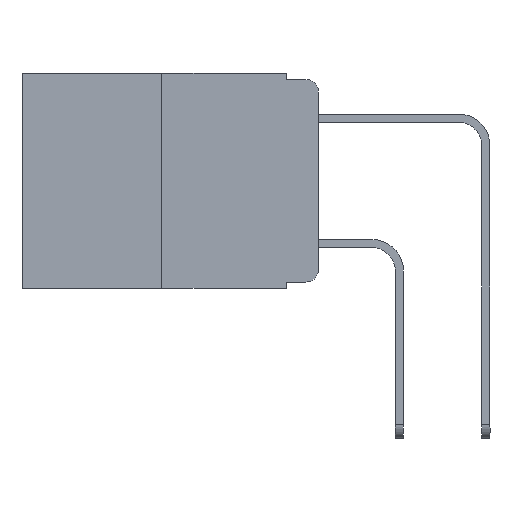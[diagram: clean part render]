
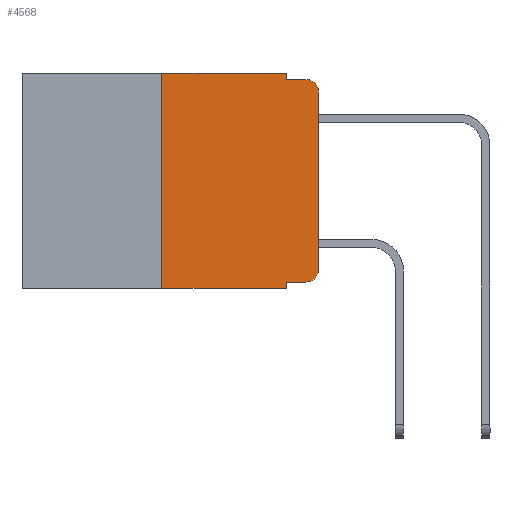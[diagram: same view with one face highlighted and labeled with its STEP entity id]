
A CAD part, left-side view. The second image highlights one B-rep face of the part: STEP entity #4568.
In plain terms, the highlighted planar face has unit normal (-1, 0, 0).
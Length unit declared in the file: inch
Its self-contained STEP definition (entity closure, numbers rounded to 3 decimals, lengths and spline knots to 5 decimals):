
#183 = ORIENTED_EDGE ( 'NONE', *, *, #6153, .F. ) ;
#1102 = CARTESIAN_POINT ( 'NONE',  ( 0., 0.051, -0.333 ) ) ;
#1154 = EDGE_CURVE ( 'NONE', #12393, #10170, #1194, .T. ) ;
#1194 = LINE ( 'NONE', #10466, #10949 ) ;
#1299 = DIRECTION ( 'NONE',  ( 0., 0., -1. ) ) ;
#1420 = ORIENTED_EDGE ( 'NONE', *, *, #4232, .T. ) ;
#1566 = FACE_OUTER_BOUND ( 'NONE', #10264, .T. ) ;
#1589 = AXIS2_PLACEMENT_3D ( 'NONE', #11448, #7667, #1299 ) ;
#1647 = CARTESIAN_POINT ( 'NONE',  ( 0., 0.02, -0.01 ) ) ;
#2068 = CARTESIAN_POINT ( 'NONE',  ( 0., 0.051, 0. ) ) ;
#2084 = EDGE_CURVE ( 'NONE', #12351, #12169, #6772, .T. ) ;
#2119 = VECTOR ( 'NONE', #5809, 39.37008 ) ;
#2302 = ORIENTED_EDGE ( 'NONE', *, *, #6197, .T. ) ;
#2323 = VECTOR ( 'NONE', #10333, 39.37008 ) ;
#2584 = ORIENTED_EDGE ( 'NONE', *, *, #8001, .T. ) ;
#2593 = DIRECTION ( 'NONE',  ( 0., 0., -1. ) ) ;
#2973 = ORIENTED_EDGE ( 'NONE', *, *, #6102, .T. ) ;
#3120 = CIRCLE ( 'NONE', #8015, 0.02 ) ;
#3357 = EDGE_CURVE ( 'NONE', #7927, #4158, #3972, .T. ) ;
#3972 = LINE ( 'NONE', #12029, #10428 ) ;
#4046 = VECTOR ( 'NONE', #10812, 39.37008 ) ;
#4158 = VERTEX_POINT ( 'NONE', #11807 ) ;
#4232 = EDGE_CURVE ( 'NONE', #13104, #12169, #13054, .T. ) ;
#4300 = DIRECTION ( 'NONE',  ( 0., 0., 1. ) ) ;
#4515 = CARTESIAN_POINT ( 'NONE',  ( 0., 0.051, -0.01 ) ) ;
#4538 = PLANE ( 'NONE',  #9386 ) ;
#4568 = ADVANCED_FACE ( 'NONE', ( #1566 ), #4538, .F. ) ;
#4780 = LINE ( 'NONE', #11014, #6780 ) ;
#5189 = DIRECTION ( 'NONE',  ( 0., -1., 0. ) ) ;
#5514 = CARTESIAN_POINT ( 'NONE',  ( 0., 0.02, -0.313 ) ) ;
#5528 = CARTESIAN_POINT ( 'NONE',  ( 0., 0.473, 0. ) ) ;
#5641 = ORIENTED_EDGE ( 'NONE', *, *, #3357, .F. ) ;
#5809 = DIRECTION ( 'NONE',  ( 0., -1., 0. ) ) ;
#5896 = CARTESIAN_POINT ( 'NONE',  ( 0., 0.051, -0.343 ) ) ;
#5912 = DIRECTION ( 'NONE',  ( 0., 0., 1. ) ) ;
#5971 = DIRECTION ( 'NONE',  ( 0., -1., 0. ) ) ;
#6089 = LINE ( 'NONE', #2068, #2323 ) ;
#6102 = EDGE_CURVE ( 'NONE', #12351, #8554, #6208, .T. ) ;
#6153 = EDGE_CURVE ( 'NONE', #12072, #8791, #9523, .T. ) ;
#6197 = EDGE_CURVE ( 'NONE', #10170, #8791, #6734, .T. ) ;
#6208 = LINE ( 'NONE', #1102, #7807 ) ;
#6734 = CIRCLE ( 'NONE', #1589, 0.02 ) ;
#6772 = LINE ( 'NONE', #7728, #4046 ) ;
#6780 = VECTOR ( 'NONE', #5912, 39.37008 ) ;
#7667 = DIRECTION ( 'NONE',  ( -1., 0., 0. ) ) ;
#7728 = CARTESIAN_POINT ( 'NONE',  ( 0., 0.051, 0. ) ) ;
#7807 = VECTOR ( 'NONE', #5189, 39.37008 ) ;
#7927 = VERTEX_POINT ( 'NONE', #9189 ) ;
#7992 = ORIENTED_EDGE ( 'NONE', *, *, #10479, .F. ) ;
#8001 = EDGE_CURVE ( 'NONE', #8554, #12393, #3120, .T. ) ;
#8015 = AXIS2_PLACEMENT_3D ( 'NONE', #5514, #9576, #12445 ) ;
#8400 = CARTESIAN_POINT ( 'NONE',  ( 0., 0.051, -0.01 ) ) ;
#8554 = VERTEX_POINT ( 'NONE', #8833 ) ;
#8561 = ORIENTED_EDGE ( 'NONE', *, *, #2084, .F. ) ;
#8604 = DIRECTION ( 'NONE',  ( 1., 0., 0. ) ) ;
#8791 = VERTEX_POINT ( 'NONE', #1647 ) ;
#8833 = CARTESIAN_POINT ( 'NONE',  ( 0., 0.02, -0.333 ) ) ;
#8971 = CARTESIAN_POINT ( 'NONE',  ( 0., 0.25, -0.343 ) ) ;
#9189 = CARTESIAN_POINT ( 'NONE',  ( 0., 0.25, 0. ) ) ;
#9219 = CARTESIAN_POINT ( 'NONE',  ( 0., 0.051, -0.333 ) ) ;
#9386 = AXIS2_PLACEMENT_3D ( 'NONE', #5528, #8604, #2593 ) ;
#9523 = LINE ( 'NONE', #8400, #12884 ) ;
#9576 = DIRECTION ( 'NONE',  ( -1., 0., 0. ) ) ;
#9932 = CARTESIAN_POINT ( 'NONE',  ( 0., 0.473, -0.343 ) ) ;
#10170 = VERTEX_POINT ( 'NONE', #10299 ) ;
#10264 = EDGE_LOOP ( 'NONE', ( #11466, #2302, #183, #11674, #5641, #7992, #1420, #8561, #2973, #2584 ) ) ;
#10299 = CARTESIAN_POINT ( 'NONE',  ( 0., 0., -0.03 ) ) ;
#10333 = DIRECTION ( 'NONE',  ( 0., 0., -1. ) ) ;
#10428 = VECTOR ( 'NONE', #5971, 39.37008 ) ;
#10466 = CARTESIAN_POINT ( 'NONE',  ( 0., 0., 0. ) ) ;
#10479 = EDGE_CURVE ( 'NONE', #13104, #7927, #4780, .T. ) ;
#10812 = DIRECTION ( 'NONE',  ( 0., 0., -1. ) ) ;
#10949 = VECTOR ( 'NONE', #4300, 39.37008 ) ;
#11014 = CARTESIAN_POINT ( 'NONE',  ( 0., 0.25, 0. ) ) ;
#11046 = EDGE_CURVE ( 'NONE', #4158, #12072, #6089, .T. ) ;
#11448 = CARTESIAN_POINT ( 'NONE',  ( 0., 0.02, -0.03 ) ) ;
#11466 = ORIENTED_EDGE ( 'NONE', *, *, #1154, .T. ) ;
#11612 = CARTESIAN_POINT ( 'NONE',  ( 0., 0., -0.313 ) ) ;
#11674 = ORIENTED_EDGE ( 'NONE', *, *, #11046, .F. ) ;
#11807 = CARTESIAN_POINT ( 'NONE',  ( 0., 0.051, 0. ) ) ;
#12029 = CARTESIAN_POINT ( 'NONE',  ( 0., 0.473, 0. ) ) ;
#12072 = VERTEX_POINT ( 'NONE', #4515 ) ;
#12169 = VERTEX_POINT ( 'NONE', #5896 ) ;
#12351 = VERTEX_POINT ( 'NONE', #9219 ) ;
#12393 = VERTEX_POINT ( 'NONE', #11612 ) ;
#12445 = DIRECTION ( 'NONE',  ( 0., 0., -1. ) ) ;
#12459 = DIRECTION ( 'NONE',  ( 0., -1., 0. ) ) ;
#12884 = VECTOR ( 'NONE', #12459, 39.37008 ) ;
#13054 = LINE ( 'NONE', #9932, #2119 ) ;
#13104 = VERTEX_POINT ( 'NONE', #8971 ) ;
